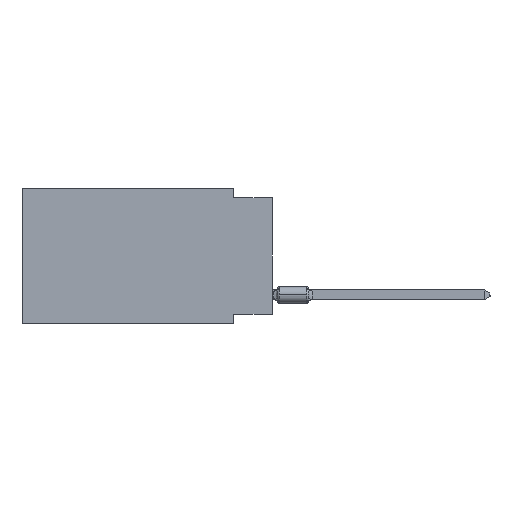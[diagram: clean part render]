
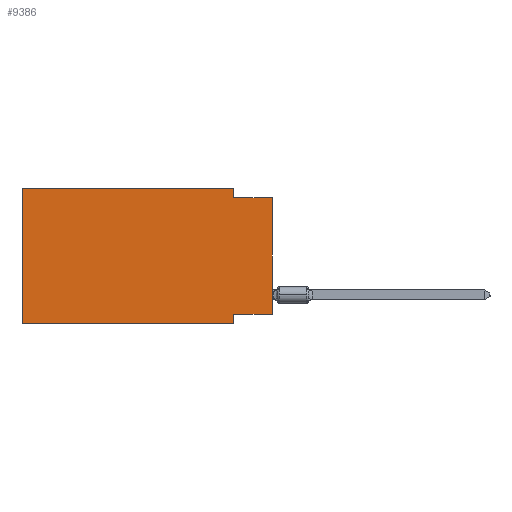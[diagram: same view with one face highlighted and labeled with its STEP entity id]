
A CAD part, left-side view. The second image highlights one B-rep face of the part: STEP entity #9386.
In plain terms, the highlighted planar face has unit normal (-1, 0, 0).
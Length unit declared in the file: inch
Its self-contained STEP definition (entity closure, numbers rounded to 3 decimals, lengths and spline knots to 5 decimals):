
#2068 = ORIENTED_EDGE ( 'NONE', *, *, #32714, .F. ) ;
#5094 = CARTESIAN_POINT ( 'NONE',  ( 0., 0.1, 0. ) ) ;
#6156 = ORIENTED_EDGE ( 'NONE', *, *, #20203, .F. ) ;
#6639 = ORIENTED_EDGE ( 'NONE', *, *, #56645, .F. ) ;
#7416 = CARTESIAN_POINT ( 'NONE',  ( 0., 0., -0.025 ) ) ;
#8842 = ORIENTED_EDGE ( 'NONE', *, *, #51179, .F. ) ;
#9386 = ADVANCED_FACE ( 'NONE', ( #50049 ), #56160, .F. ) ;
#10258 = CARTESIAN_POINT ( 'NONE',  ( 0., 0.645, 0. ) ) ;
#10802 = LINE ( 'NONE', #5094, #64412 ) ;
#13204 = DIRECTION ( 'NONE',  ( 0., 0., -1. ) ) ;
#14468 = EDGE_CURVE ( 'NONE', #22021, #46832, #31700, .T. ) ;
#16352 = CARTESIAN_POINT ( 'NONE',  ( 0., 0., 0. ) ) ;
#17451 = CARTESIAN_POINT ( 'NONE',  ( 0., 0.1, -0.325 ) ) ;
#17846 = DIRECTION ( 'NONE',  ( 1., 0., 0. ) ) ;
#18691 = CARTESIAN_POINT ( 'NONE',  ( 0., 0.1, -0.025 ) ) ;
#19645 = EDGE_CURVE ( 'NONE', #22021, #45746, #51870, .T. ) ;
#20203 = EDGE_CURVE ( 'NONE', #26131, #45746, #24665, .T. ) ;
#20577 = CARTESIAN_POINT ( 'NONE',  ( 0., 0.1, -0.35 ) ) ;
#21716 = LINE ( 'NONE', #16352, #61537 ) ;
#21857 = VECTOR ( 'NONE', #37375, 39.37008 ) ;
#22021 = VERTEX_POINT ( 'NONE', #48861 ) ;
#23177 = CARTESIAN_POINT ( 'NONE',  ( 0., 0., -0.325 ) ) ;
#23949 = DIRECTION ( 'NONE',  ( 0., -1., 0. ) ) ;
#24545 = VERTEX_POINT ( 'NONE', #61789 ) ;
#24571 = VERTEX_POINT ( 'NONE', #7416 ) ;
#24665 = LINE ( 'NONE', #20577, #21857 ) ;
#24741 = VECTOR ( 'NONE', #70565, 39.37008 ) ;
#25292 = VECTOR ( 'NONE', #48151, 39.37008 ) ;
#26131 = VERTEX_POINT ( 'NONE', #17451 ) ;
#27230 = DIRECTION ( 'NONE',  ( 0., 0., -1. ) ) ;
#28333 = ORIENTED_EDGE ( 'NONE', *, *, #63442, .T. ) ;
#31700 = LINE ( 'NONE', #10258, #59342 ) ;
#32714 = EDGE_CURVE ( 'NONE', #24545, #38349, #10802, .T. ) ;
#33686 = CARTESIAN_POINT ( 'NONE',  ( 0., 0.645, 0. ) ) ;
#33982 = ORIENTED_EDGE ( 'NONE', *, *, #19645, .T. ) ;
#37375 = DIRECTION ( 'NONE',  ( 0., 0., -1. ) ) ;
#38349 = VERTEX_POINT ( 'NONE', #18691 ) ;
#40391 = CARTESIAN_POINT ( 'NONE',  ( 0., 0.645, 0. ) ) ;
#42222 = VERTEX_POINT ( 'NONE', #23177 ) ;
#42767 = LINE ( 'NONE', #60296, #25292 ) ;
#45746 = VERTEX_POINT ( 'NONE', #64502 ) ;
#46832 = VERTEX_POINT ( 'NONE', #57427 ) ;
#47828 = DIRECTION ( 'NONE',  ( 0., 0., 1. ) ) ;
#48151 = DIRECTION ( 'NONE',  ( 0., -1., 0. ) ) ;
#48745 = EDGE_CURVE ( 'NONE', #38349, #24571, #42767, .T. ) ;
#48861 = CARTESIAN_POINT ( 'NONE',  ( 0., 0.645, -0.35 ) ) ;
#50049 = FACE_OUTER_BOUND ( 'NONE', #54585, .T. ) ;
#51179 = EDGE_CURVE ( 'NONE', #46832, #24545, #60903, .T. ) ;
#51870 = LINE ( 'NONE', #56535, #57228 ) ;
#54585 = EDGE_LOOP ( 'NONE', ( #28333, #56377, #2068, #8842, #55355, #33982, #6156, #6639 ) ) ;
#55355 = ORIENTED_EDGE ( 'NONE', *, *, #14468, .F. ) ;
#55897 = LINE ( 'NONE', #60203, #24741 ) ;
#56160 = PLANE ( 'NONE',  #66901 ) ;
#56377 = ORIENTED_EDGE ( 'NONE', *, *, #48745, .F. ) ;
#56535 = CARTESIAN_POINT ( 'NONE',  ( 0., 0.645, -0.35 ) ) ;
#56645 = EDGE_CURVE ( 'NONE', #42222, #26131, #55897, .T. ) ;
#57228 = VECTOR ( 'NONE', #23949, 39.37008 ) ;
#57427 = CARTESIAN_POINT ( 'NONE',  ( 0., 0.645, 0. ) ) ;
#59342 = VECTOR ( 'NONE', #47828, 39.37008 ) ;
#60203 = CARTESIAN_POINT ( 'NONE',  ( 0., 0., -0.325 ) ) ;
#60296 = CARTESIAN_POINT ( 'NONE',  ( 0., 0., -0.025 ) ) ;
#60903 = LINE ( 'NONE', #33686, #67857 ) ;
#61537 = VECTOR ( 'NONE', #65708, 39.37008 ) ;
#61789 = CARTESIAN_POINT ( 'NONE',  ( 0., 0.1, 0. ) ) ;
#63442 = EDGE_CURVE ( 'NONE', #42222, #24571, #21716, .T. ) ;
#63969 = DIRECTION ( 'NONE',  ( 0., -1., 0. ) ) ;
#64412 = VECTOR ( 'NONE', #27230, 39.37008 ) ;
#64502 = CARTESIAN_POINT ( 'NONE',  ( 0., 0.1, -0.35 ) ) ;
#65708 = DIRECTION ( 'NONE',  ( 0., 0., 1. ) ) ;
#66901 = AXIS2_PLACEMENT_3D ( 'NONE', #40391, #17846, #13204 ) ;
#67857 = VECTOR ( 'NONE', #63969, 39.37008 ) ;
#70565 = DIRECTION ( 'NONE',  ( 0., 1., 0. ) ) ;
